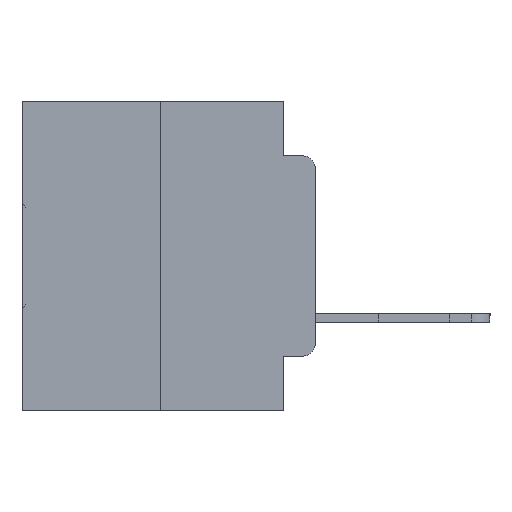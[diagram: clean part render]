
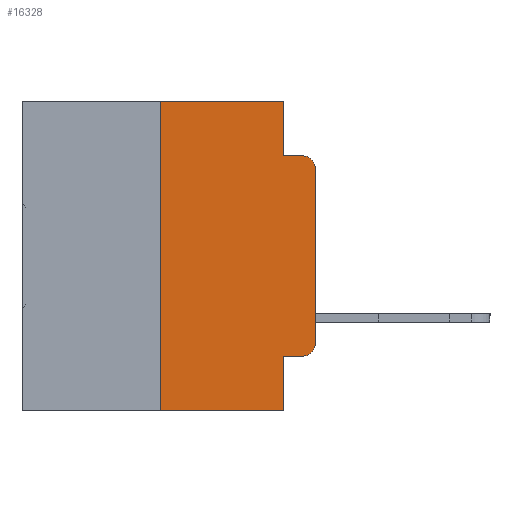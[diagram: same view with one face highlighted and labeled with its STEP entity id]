
A CAD part, left-side view. The second image highlights one B-rep face of the part: STEP entity #16328.
In plain terms, the highlighted planar face has unit normal (-1, 0, 0).
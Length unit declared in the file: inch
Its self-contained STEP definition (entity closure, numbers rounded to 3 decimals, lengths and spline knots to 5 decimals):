
#577 = VECTOR ( 'NONE', #15514, 39.37008 ) ;
#1581 = CARTESIAN_POINT ( 'NONE',  ( 0., 0.051, -0.4115 ) ) ;
#1628 = EDGE_CURVE ( 'NONE', #30611, #13405, #9497, .T. ) ;
#1816 = ORIENTED_EDGE ( 'NONE', *, *, #16638, .F. ) ;
#1941 = LINE ( 'NONE', #14679, #26409 ) ;
#1968 = VERTEX_POINT ( 'NONE', #7279 ) ;
#2019 = CARTESIAN_POINT ( 'NONE',  ( 0., 0.051, 0. ) ) ;
#2170 = ORIENTED_EDGE ( 'NONE', *, *, #2815, .T. ) ;
#2424 = EDGE_CURVE ( 'NONE', #23953, #7845, #4613, .T. ) ;
#2803 = CARTESIAN_POINT ( 'NONE',  ( 0., 0.02, -0.0885 ) ) ;
#2815 = EDGE_CURVE ( 'NONE', #13405, #1968, #12411, .T. ) ;
#2863 = DIRECTION ( 'NONE',  ( 0., -1., 0. ) ) ;
#3612 = ORIENTED_EDGE ( 'NONE', *, *, #27236, .T. ) ;
#3959 = CARTESIAN_POINT ( 'NONE',  ( 0., 0.473, -0.5 ) ) ;
#4613 = LINE ( 'NONE', #9559, #10947 ) ;
#4720 = DIRECTION ( 'NONE',  ( 0., -1., 0. ) ) ;
#4767 = VECTOR ( 'NONE', #23176, 39.37008 ) ;
#5062 = VECTOR ( 'NONE', #11688, 39.37008 ) ;
#5569 = CARTESIAN_POINT ( 'NONE',  ( 0., 0.25, -0.5 ) ) ;
#6359 = DIRECTION ( 'NONE',  ( 0., -1., 0. ) ) ;
#6880 = CARTESIAN_POINT ( 'NONE',  ( 0., 0.02, -0.4115 ) ) ;
#7002 = ORIENTED_EDGE ( 'NONE', *, *, #13125, .F. ) ;
#7279 = CARTESIAN_POINT ( 'NONE',  ( 0., 0., -0.1085 ) ) ;
#7469 = DIRECTION ( 'NONE',  ( -1., 0., 0. ) ) ;
#7845 = VERTEX_POINT ( 'NONE', #9928 ) ;
#9303 = EDGE_LOOP ( 'NONE', ( #2170, #3612, #29576, #17762, #1816, #16641, #29231, #7002, #15535, #30327 ) ) ;
#9497 = CIRCLE ( 'NONE', #23706, 0.02 ) ;
#9559 = CARTESIAN_POINT ( 'NONE',  ( 0., 0.051, 0. ) ) ;
#9766 = EDGE_CURVE ( 'NONE', #7845, #21079, #1941, .T. ) ;
#9895 = LINE ( 'NONE', #30584, #5062 ) ;
#9928 = CARTESIAN_POINT ( 'NONE',  ( 0., 0.051, -0.0885 ) ) ;
#10305 = AXIS2_PLACEMENT_3D ( 'NONE', #21733, #7469, #24092 ) ;
#10798 = VERTEX_POINT ( 'NONE', #25927 ) ;
#10866 = AXIS2_PLACEMENT_3D ( 'NONE', #22087, #12612, #29158 ) ;
#10947 = VECTOR ( 'NONE', #16173, 39.37008 ) ;
#11688 = DIRECTION ( 'NONE',  ( 0., 0., 1. ) ) ;
#12411 = LINE ( 'NONE', #15380, #577 ) ;
#12554 = EDGE_CURVE ( 'NONE', #29703, #21861, #9895, .T. ) ;
#12612 = DIRECTION ( 'NONE',  ( 1., 0., 0. ) ) ;
#12825 = CARTESIAN_POINT ( 'NONE',  ( 0., 0.25, 0. ) ) ;
#13125 = EDGE_CURVE ( 'NONE', #13598, #10798, #24305, .T. ) ;
#13405 = VERTEX_POINT ( 'NONE', #26746 ) ;
#13598 = VERTEX_POINT ( 'NONE', #1581 ) ;
#13612 = CARTESIAN_POINT ( 'NONE',  ( 0., 0.473, 0. ) ) ;
#14669 = EDGE_CURVE ( 'NONE', #29703, #10798, #16752, .T. ) ;
#14679 = CARTESIAN_POINT ( 'NONE',  ( 0., 0.051, -0.0885 ) ) ;
#15380 = CARTESIAN_POINT ( 'NONE',  ( 0., 0., 0. ) ) ;
#15514 = DIRECTION ( 'NONE',  ( 0., 0., 1. ) ) ;
#15535 = ORIENTED_EDGE ( 'NONE', *, *, #18524, .T. ) ;
#16040 = DIRECTION ( 'NONE',  ( 0., 0., -1. ) ) ;
#16173 = DIRECTION ( 'NONE',  ( 0., 0., -1. ) ) ;
#16328 = ADVANCED_FACE ( 'NONE', ( #26329 ), #26806, .F. ) ;
#16638 = EDGE_CURVE ( 'NONE', #21861, #23953, #18173, .T. ) ;
#16641 = ORIENTED_EDGE ( 'NONE', *, *, #12554, .F. ) ;
#16752 = LINE ( 'NONE', #3959, #22351 ) ;
#16871 = DIRECTION ( 'NONE',  ( -1., 0., 0. ) ) ;
#17040 = CARTESIAN_POINT ( 'NONE',  ( 0., 0.02, -0.3915 ) ) ;
#17762 = ORIENTED_EDGE ( 'NONE', *, *, #2424, .F. ) ;
#18173 = LINE ( 'NONE', #13612, #4767 ) ;
#18524 = EDGE_CURVE ( 'NONE', #13598, #30611, #20660, .T. ) ;
#18763 = VECTOR ( 'NONE', #23358, 39.37008 ) ;
#19937 = VECTOR ( 'NONE', #4720, 39.37008 ) ;
#20660 = LINE ( 'NONE', #28356, #19937 ) ;
#21079 = VERTEX_POINT ( 'NONE', #2803 ) ;
#21733 = CARTESIAN_POINT ( 'NONE',  ( 0., 0.02, -0.1085 ) ) ;
#21861 = VERTEX_POINT ( 'NONE', #12825 ) ;
#22087 = CARTESIAN_POINT ( 'NONE',  ( 0., 0.473, 0. ) ) ;
#22351 = VECTOR ( 'NONE', #6359, 39.37008 ) ;
#23176 = DIRECTION ( 'NONE',  ( 0., -1., 0. ) ) ;
#23358 = DIRECTION ( 'NONE',  ( 0., 0., -1. ) ) ;
#23706 = AXIS2_PLACEMENT_3D ( 'NONE', #17040, #16871, #16040 ) ;
#23953 = VERTEX_POINT ( 'NONE', #27908 ) ;
#24092 = DIRECTION ( 'NONE',  ( 0., 0., -1. ) ) ;
#24305 = LINE ( 'NONE', #2019, #18763 ) ;
#24832 = CIRCLE ( 'NONE', #10305, 0.02 ) ;
#25927 = CARTESIAN_POINT ( 'NONE',  ( 0., 0.051, -0.5 ) ) ;
#26329 = FACE_OUTER_BOUND ( 'NONE', #9303, .T. ) ;
#26409 = VECTOR ( 'NONE', #2863, 39.37008 ) ;
#26746 = CARTESIAN_POINT ( 'NONE',  ( 0., 0., -0.3915 ) ) ;
#26806 = PLANE ( 'NONE',  #10866 ) ;
#27236 = EDGE_CURVE ( 'NONE', #1968, #21079, #24832, .T. ) ;
#27908 = CARTESIAN_POINT ( 'NONE',  ( 0., 0.051, 0. ) ) ;
#28356 = CARTESIAN_POINT ( 'NONE',  ( 0., 0.051, -0.4115 ) ) ;
#29158 = DIRECTION ( 'NONE',  ( 0., 0., -1. ) ) ;
#29231 = ORIENTED_EDGE ( 'NONE', *, *, #14669, .T. ) ;
#29576 = ORIENTED_EDGE ( 'NONE', *, *, #9766, .F. ) ;
#29703 = VERTEX_POINT ( 'NONE', #5569 ) ;
#30327 = ORIENTED_EDGE ( 'NONE', *, *, #1628, .T. ) ;
#30584 = CARTESIAN_POINT ( 'NONE',  ( 0., 0.25, 0. ) ) ;
#30611 = VERTEX_POINT ( 'NONE', #6880 ) ;
